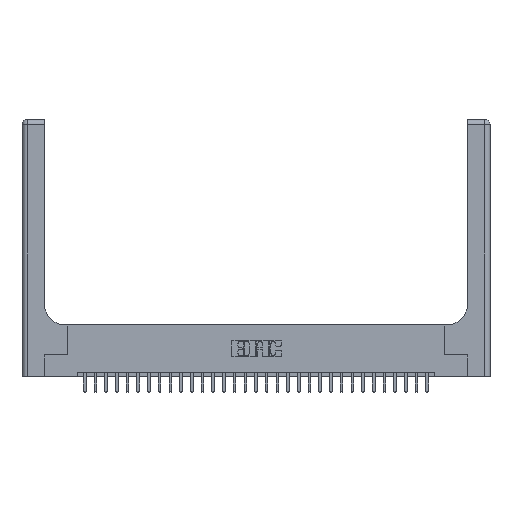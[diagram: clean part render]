
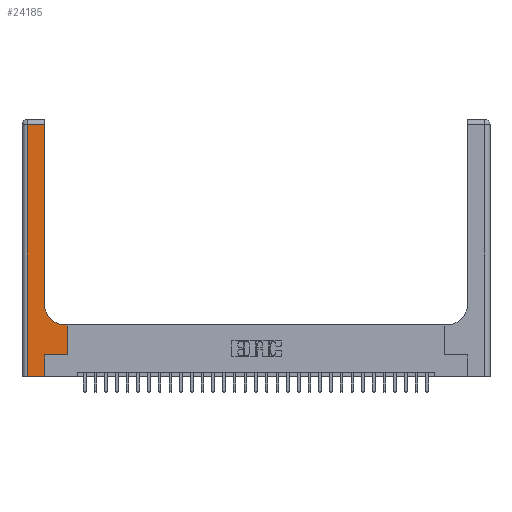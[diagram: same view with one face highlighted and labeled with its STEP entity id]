
A CAD part, top view. The second image highlights one B-rep face of the part: STEP entity #24185.
In plain terms, the highlighted planar face has unit normal (0, 0, 1).
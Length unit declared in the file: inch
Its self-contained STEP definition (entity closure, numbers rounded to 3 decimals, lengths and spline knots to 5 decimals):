
#42 = LINE ( 'NONE', #4219, #21748 ) ;
#167 = EDGE_CURVE ( 'NONE', #10450, #2218, #19986, .T. ) ;
#247 = DIRECTION ( 'NONE',  ( 1., 0., 0. ) ) ;
#644 = VERTEX_POINT ( 'NONE', #22084 ) ;
#1333 = ORIENTED_EDGE ( 'NONE', *, *, #25245, .T. ) ;
#2112 = VERTEX_POINT ( 'NONE', #25296 ) ;
#2218 = VERTEX_POINT ( 'NONE', #23409 ) ;
#2871 = AXIS2_PLACEMENT_3D ( 'NONE', #26489, #19863, #247 ) ;
#3420 = ORIENTED_EDGE ( 'NONE', *, *, #5577, .T. ) ;
#3674 = LINE ( 'NONE', #18800, #19079 ) ;
#3948 = CARTESIAN_POINT ( 'NONE',  ( 0.26, 0.6, 0.37 ) ) ;
#4032 = DIRECTION ( 'NONE',  ( 1., 0., 0. ) ) ;
#4219 = CARTESIAN_POINT ( 'NONE',  ( 0., 2.94, 0.37 ) ) ;
#4579 = EDGE_CURVE ( 'NONE', #21993, #5743, #11613, .T. ) ;
#4797 = DIRECTION ( 'NONE',  ( 1., 0., 0. ) ) ;
#4858 = DIRECTION ( 'NONE',  ( 0., 1., 0. ) ) ;
#5023 = VECTOR ( 'NONE', #27866, 39.37008 ) ;
#5098 = LINE ( 'NONE', #22665, #10281 ) ;
#5487 = ORIENTED_EDGE ( 'NONE', *, *, #167, .T. ) ;
#5577 = EDGE_CURVE ( 'NONE', #28407, #2112, #15138, .T. ) ;
#5743 = VERTEX_POINT ( 'NONE', #15834 ) ;
#6073 = DIRECTION ( 'NONE',  ( -1., 0., 0. ) ) ;
#7379 = EDGE_CURVE ( 'NONE', #644, #21993, #7897, .T. ) ;
#7897 = CIRCLE ( 'NONE', #2871, 0.25 ) ;
#8079 = EDGE_CURVE ( 'NONE', #2112, #644, #19083, .T. ) ;
#8807 = DIRECTION ( 'NONE',  ( -1., 0., 0. ) ) ;
#8877 = ORIENTED_EDGE ( 'NONE', *, *, #18343, .T. ) ;
#9435 = CARTESIAN_POINT ( 'NONE',  ( 0.26, 3., 0.37 ) ) ;
#9843 = VECTOR ( 'NONE', #26621, 39.37008 ) ;
#9849 = AXIS2_PLACEMENT_3D ( 'NONE', #10374, #25830, #6073 ) ;
#10154 = CARTESIAN_POINT ( 'NONE',  ( 0.26, 0.85, 0.37 ) ) ;
#10281 = VECTOR ( 'NONE', #4797, 39.37008 ) ;
#10374 = CARTESIAN_POINT ( 'NONE',  ( 0., 3., 0.37 ) ) ;
#10450 = VERTEX_POINT ( 'NONE', #24017 ) ;
#10573 = ORIENTED_EDGE ( 'NONE', *, *, #8079, .T. ) ;
#10716 = ORIENTED_EDGE ( 'NONE', *, *, #26408, .T. ) ;
#10882 = EDGE_LOOP ( 'NONE', ( #22306, #10716, #5487, #1333, #8877, #26678, #3420, #10573, #16215 ) ) ;
#11613 = LINE ( 'NONE', #9435, #5023 ) ;
#11766 = EDGE_CURVE ( 'NONE', #27534, #28407, #25938, .T. ) ;
#11800 = CARTESIAN_POINT ( 'NONE',  ( 0.528, 0.25, 0.37 ) ) ;
#12953 = PLANE ( 'NONE',  #9849 ) ;
#15132 = VECTOR ( 'NONE', #23942, 39.37008 ) ;
#15138 = LINE ( 'NONE', #19331, #15132 ) ;
#15713 = CARTESIAN_POINT ( 'NONE',  ( 0.265, 0., 0.37 ) ) ;
#15834 = CARTESIAN_POINT ( 'NONE',  ( 0.26, 2.94, 0.37 ) ) ;
#16215 = ORIENTED_EDGE ( 'NONE', *, *, #7379, .T. ) ;
#16738 = FACE_OUTER_BOUND ( 'NONE', #10882, .T. ) ;
#18343 = EDGE_CURVE ( 'NONE', #19125, #27534, #3674, .T. ) ;
#18800 = CARTESIAN_POINT ( 'NONE',  ( 0.265, 0., 0.37 ) ) ;
#19079 = VECTOR ( 'NONE', #4858, 39.37008 ) ;
#19083 = LINE ( 'NONE', #3948, #26382 ) ;
#19125 = VERTEX_POINT ( 'NONE', #15713 ) ;
#19331 = CARTESIAN_POINT ( 'NONE',  ( 0.528, 0.25, 0.37 ) ) ;
#19863 = DIRECTION ( 'NONE',  ( 0., 0., -1. ) ) ;
#19986 = LINE ( 'NONE', #24454, #9843 ) ;
#21748 = VECTOR ( 'NONE', #8807, 39.37008 ) ;
#21993 = VERTEX_POINT ( 'NONE', #10154 ) ;
#22084 = CARTESIAN_POINT ( 'NONE',  ( 0.51, 0.6, 0.37 ) ) ;
#22306 = ORIENTED_EDGE ( 'NONE', *, *, #4579, .T. ) ;
#22665 = CARTESIAN_POINT ( 'NONE',  ( 0., 0., 0.37 ) ) ;
#23409 = CARTESIAN_POINT ( 'NONE',  ( 0.06, 0., 0.37 ) ) ;
#23773 = CARTESIAN_POINT ( 'NONE',  ( 0.265, 0.25, 0.37 ) ) ;
#23942 = DIRECTION ( 'NONE',  ( 0., 1., 0. ) ) ;
#24017 = CARTESIAN_POINT ( 'NONE',  ( 0.06, 2.94, 0.37 ) ) ;
#24185 = ADVANCED_FACE ( 'NONE', ( #16738 ), #12953, .F. ) ;
#24454 = CARTESIAN_POINT ( 'NONE',  ( 0.06, 3., 0.37 ) ) ;
#25245 = EDGE_CURVE ( 'NONE', #2218, #19125, #5098, .T. ) ;
#25296 = CARTESIAN_POINT ( 'NONE',  ( 0.528, 0.6, 0.37 ) ) ;
#25830 = DIRECTION ( 'NONE',  ( 0., 0., -1. ) ) ;
#25938 = LINE ( 'NONE', #23773, #26141 ) ;
#26141 = VECTOR ( 'NONE', #4032, 39.37008 ) ;
#26382 = VECTOR ( 'NONE', #27876, 39.37008 ) ;
#26408 = EDGE_CURVE ( 'NONE', #5743, #10450, #42, .T. ) ;
#26489 = CARTESIAN_POINT ( 'NONE',  ( 0.51, 0.85, 0.37 ) ) ;
#26621 = DIRECTION ( 'NONE',  ( 0., -1., 0. ) ) ;
#26678 = ORIENTED_EDGE ( 'NONE', *, *, #11766, .T. ) ;
#27534 = VERTEX_POINT ( 'NONE', #27875 ) ;
#27866 = DIRECTION ( 'NONE',  ( 0., 1., 0. ) ) ;
#27875 = CARTESIAN_POINT ( 'NONE',  ( 0.265, 0.25, 0.37 ) ) ;
#27876 = DIRECTION ( 'NONE',  ( -1., 0., 0. ) ) ;
#28407 = VERTEX_POINT ( 'NONE', #11800 ) ;
